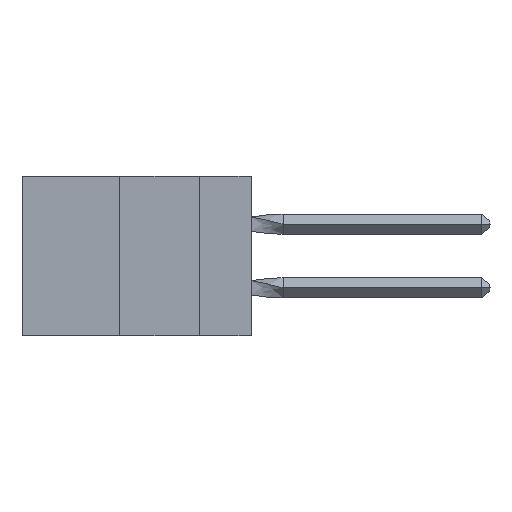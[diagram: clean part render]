
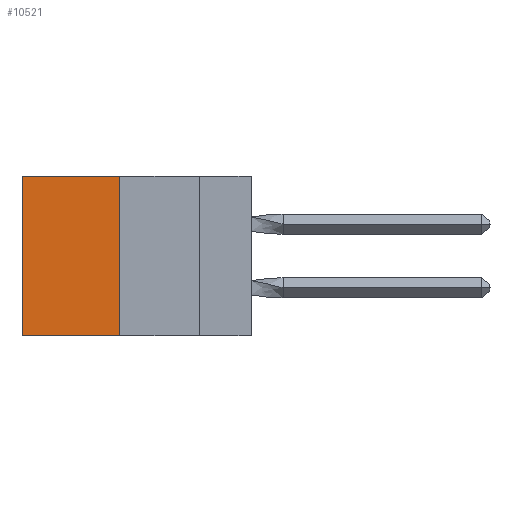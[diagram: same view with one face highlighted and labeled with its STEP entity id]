
A CAD part, left-side view. The second image highlights one B-rep face of the part: STEP entity #10521.
In plain terms, the highlighted planar face has unit normal (-1, 0, 0).
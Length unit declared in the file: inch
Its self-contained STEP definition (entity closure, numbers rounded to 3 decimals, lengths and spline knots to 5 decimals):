
#445 = LINE ( 'NONE', #31718, #33806 ) ;
#482 = VERTEX_POINT ( 'NONE', #38383 ) ;
#768 = EDGE_LOOP ( 'NONE', ( #27808, #31508, #29155, #35200 ) ) ;
#1474 = VERTEX_POINT ( 'NONE', #3557 ) ;
#2062 = LINE ( 'NONE', #4334, #24785 ) ;
#2074 = DIRECTION ( 'NONE',  ( 0., 0., -1. ) ) ;
#2972 = CARTESIAN_POINT ( 'NONE',  ( 0.305, 0.413, -0.5 ) ) ;
#3124 = VECTOR ( 'NONE', #5744, 39.37008 ) ;
#3557 = CARTESIAN_POINT ( 'NONE',  ( 0.305, 0.72, -0.5 ) ) ;
#4334 = CARTESIAN_POINT ( 'NONE',  ( 0.305, 0.413, 0. ) ) ;
#5744 = DIRECTION ( 'NONE',  ( 0., 1., 0. ) ) ;
#6573 = EDGE_CURVE ( 'NONE', #482, #25422, #2062, .T. ) ;
#6726 = PLANE ( 'NONE',  #27468 ) ;
#7350 = CARTESIAN_POINT ( 'NONE',  ( 0.305, 0.413, -0.5 ) ) ;
#10189 = EDGE_CURVE ( 'NONE', #25422, #1474, #445, .T. ) ;
#10521 = ADVANCED_FACE ( 'NONE', ( #23091 ), #6726, .F. ) ;
#10991 = VERTEX_POINT ( 'NONE', #2972 ) ;
#12596 = DIRECTION ( 'NONE',  ( 0., 1., 0. ) ) ;
#13189 = DIRECTION ( 'NONE',  ( 1., 0., 0. ) ) ;
#13647 = EDGE_CURVE ( 'NONE', #482, #10991, #24768, .T. ) ;
#22097 = CARTESIAN_POINT ( 'NONE',  ( 0.305, 0.72, 0. ) ) ;
#23091 = FACE_OUTER_BOUND ( 'NONE', #768, .T. ) ;
#24768 = LINE ( 'NONE', #7350, #27969 ) ;
#24785 = VECTOR ( 'NONE', #12596, 39.37008 ) ;
#25207 = DIRECTION ( 'NONE',  ( 0., 0., -1. ) ) ;
#25422 = VERTEX_POINT ( 'NONE', #22097 ) ;
#27247 = EDGE_CURVE ( 'NONE', #10991, #1474, #35974, .T. ) ;
#27411 = CARTESIAN_POINT ( 'NONE',  ( 0.305, 0.413, -0.5 ) ) ;
#27468 = AXIS2_PLACEMENT_3D ( 'NONE', #27411, #13189, #33885 ) ;
#27808 = ORIENTED_EDGE ( 'NONE', *, *, #10189, .T. ) ;
#27969 = VECTOR ( 'NONE', #25207, 39.37008 ) ;
#29155 = ORIENTED_EDGE ( 'NONE', *, *, #13647, .F. ) ;
#31508 = ORIENTED_EDGE ( 'NONE', *, *, #27247, .F. ) ;
#31718 = CARTESIAN_POINT ( 'NONE',  ( 0.305, 0.72, -0.5 ) ) ;
#33806 = VECTOR ( 'NONE', #2074, 39.37008 ) ;
#33885 = DIRECTION ( 'NONE',  ( 0., 0., -1. ) ) ;
#35200 = ORIENTED_EDGE ( 'NONE', *, *, #6573, .T. ) ;
#35246 = CARTESIAN_POINT ( 'NONE',  ( 0.305, 0.413, -0.5 ) ) ;
#35974 = LINE ( 'NONE', #35246, #3124 ) ;
#38383 = CARTESIAN_POINT ( 'NONE',  ( 0.305, 0.413, 0. ) ) ;
